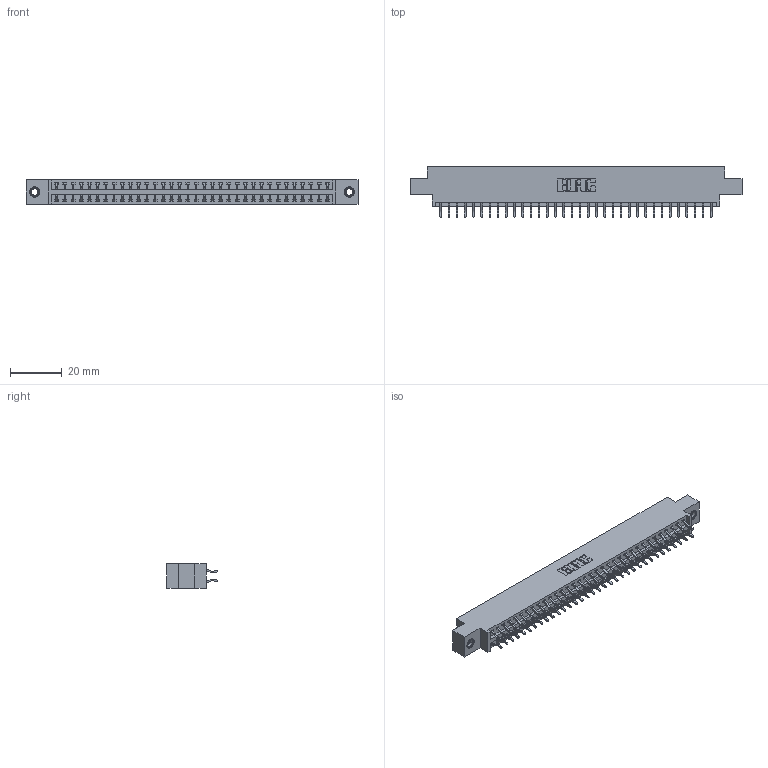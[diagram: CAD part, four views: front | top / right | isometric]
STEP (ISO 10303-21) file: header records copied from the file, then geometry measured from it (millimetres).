
FILE_DESCRIPTION (( 'STEP AP203' ), '1' );
FILE_NAME ('346-068-556-807.STEP', '2022-05-24T19:54:49', ( '' ), ( '' ), 'SwSTEP 2.0', 'SolidWorks 2020', '' );
FILE_SCHEMA (( 'CONFIG_CONTROL_DESIGN' ));
Length unit declared in the file: inch
Products named in the file (4): 345-250-001_345-250-005-103; 346-068-556-807; 345-292-001_556 Tail; 346 Part_0.170 Offset - 0.156 Dia-TI
Assembly tree (71 placements, depth 2):
  346-068-556-807
    346 Part_0.170 Offset - 0.156 Dia-TI
    345-292-001_556 Tail  x68
    345-250-001_345-250-005-103  x2
Bounding box: 128.52 x 19.57 x 9.4 mm (x, y, z)
Volume: 12299.7 mm3; surface area: 16931.3 mm2
Topology: 71 solids, 71 shells, 4130 faces, 12241 edges, 8062 vertices
Faces by surface type: plane 2764, cylinder 1350, cone 12, torus 4
Entity records: 24804 total; most frequent: CARTESIAN_POINT 4099, ORIENTED_EDGE 4014, DIRECTION 3677, EDGE_CURVE 2007, LINE 1711, VECTOR 1711, VERTEX_POINT 1332, AXIS2_PLACEMENT_3D 983
